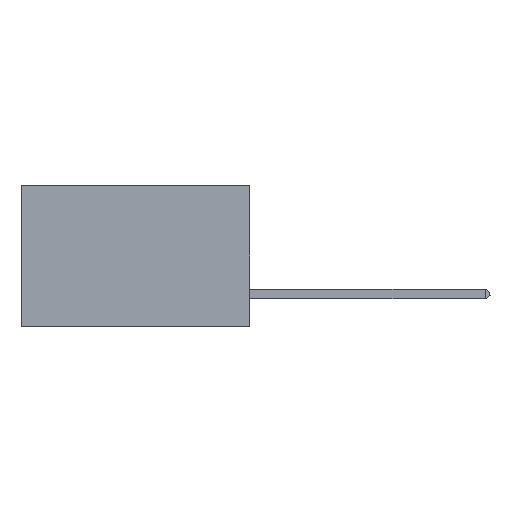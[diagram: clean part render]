
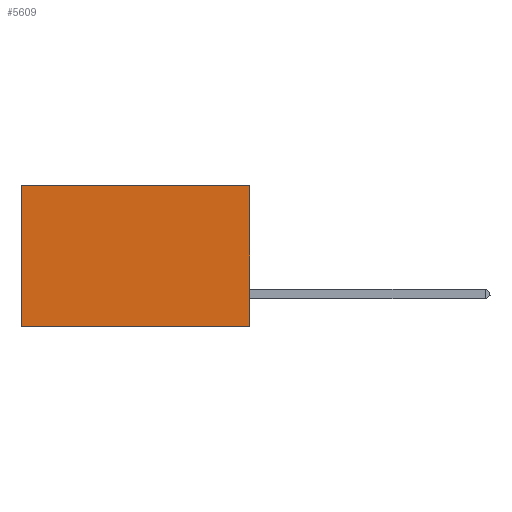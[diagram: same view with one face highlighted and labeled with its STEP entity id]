
A CAD part, left-side view. The second image highlights one B-rep face of the part: STEP entity #5609.
In plain terms, the highlighted planar face has unit normal (-1, 0, 0).
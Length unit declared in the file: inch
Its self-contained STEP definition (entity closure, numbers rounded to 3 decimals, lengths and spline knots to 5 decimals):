
#26 = EDGE_CURVE ( 'NONE', #5001, #547, #10706, .T. ) ;
#94 = CARTESIAN_POINT ( 'NONE',  ( 0.2875, 0., 0. ) ) ;
#176 = DIRECTION ( 'NONE',  ( 0., 1., 0. ) ) ;
#241 = ORIENTED_EDGE ( 'NONE', *, *, #3679, .F. ) ;
#354 = ORIENTED_EDGE ( 'NONE', *, *, #11058, .F. ) ;
#547 = VERTEX_POINT ( 'NONE', #9886 ) ;
#596 = DIRECTION ( 'NONE',  ( 1., 0., 0. ) ) ;
#637 = EDGE_CURVE ( 'NONE', #547, #8849, #7875, .T. ) ;
#2078 = CARTESIAN_POINT ( 'NONE',  ( 0.2875, 0., -0.37 ) ) ;
#2889 = CARTESIAN_POINT ( 'NONE',  ( 0.2875, 0.6, 0. ) ) ;
#3108 = VERTEX_POINT ( 'NONE', #2078 ) ;
#3450 = AXIS2_PLACEMENT_3D ( 'NONE', #9008, #596, #9041 ) ;
#3679 = EDGE_CURVE ( 'NONE', #3108, #8849, #10436, .T. ) ;
#3754 = CARTESIAN_POINT ( 'NONE',  ( 0.2875, 0., -0.37 ) ) ;
#3793 = DIRECTION ( 'NONE',  ( 0., 0., -1. ) ) ;
#3922 = LINE ( 'NONE', #4120, #10386 ) ;
#4008 = ORIENTED_EDGE ( 'NONE', *, *, #26, .T. ) ;
#4120 = CARTESIAN_POINT ( 'NONE',  ( 0.2875, 0., 0. ) ) ;
#4223 = VECTOR ( 'NONE', #176, 39.37008 ) ;
#5001 = VERTEX_POINT ( 'NONE', #9436 ) ;
#5609 = ADVANCED_FACE ( 'NONE', ( #9090 ), #7164, .F. ) ;
#5978 = VECTOR ( 'NONE', #3793, 39.37008 ) ;
#7164 = PLANE ( 'NONE',  #3450 ) ;
#7808 = EDGE_LOOP ( 'NONE', ( #7914, #241, #354, #4008 ) ) ;
#7848 = DIRECTION ( 'NONE',  ( 0., 0., -1. ) ) ;
#7875 = LINE ( 'NONE', #2889, #5978 ) ;
#7914 = ORIENTED_EDGE ( 'NONE', *, *, #637, .T. ) ;
#8828 = VECTOR ( 'NONE', #11447, 39.37008 ) ;
#8849 = VERTEX_POINT ( 'NONE', #12200 ) ;
#9008 = CARTESIAN_POINT ( 'NONE',  ( 0.2875, 0., 0. ) ) ;
#9041 = DIRECTION ( 'NONE',  ( 0., 0., -1. ) ) ;
#9090 = FACE_OUTER_BOUND ( 'NONE', #7808, .T. ) ;
#9436 = CARTESIAN_POINT ( 'NONE',  ( 0.2875, 0., 0. ) ) ;
#9886 = CARTESIAN_POINT ( 'NONE',  ( 0.2875, 0.6, 0. ) ) ;
#10386 = VECTOR ( 'NONE', #7848, 39.37008 ) ;
#10436 = LINE ( 'NONE', #3754, #8828 ) ;
#10706 = LINE ( 'NONE', #94, #4223 ) ;
#11058 = EDGE_CURVE ( 'NONE', #5001, #3108, #3922, .T. ) ;
#11447 = DIRECTION ( 'NONE',  ( 0., 1., 0. ) ) ;
#12200 = CARTESIAN_POINT ( 'NONE',  ( 0.2875, 0.6, -0.37 ) ) ;
